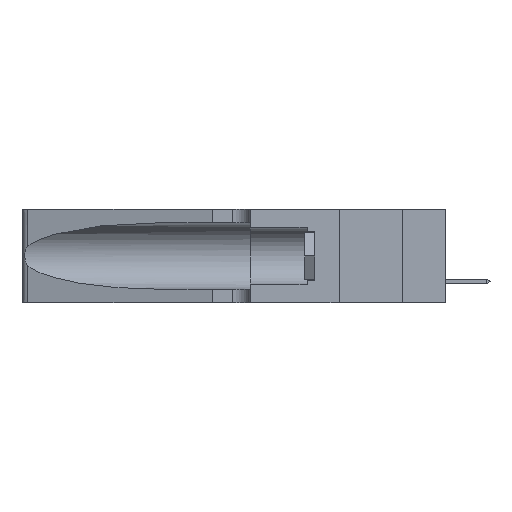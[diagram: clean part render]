
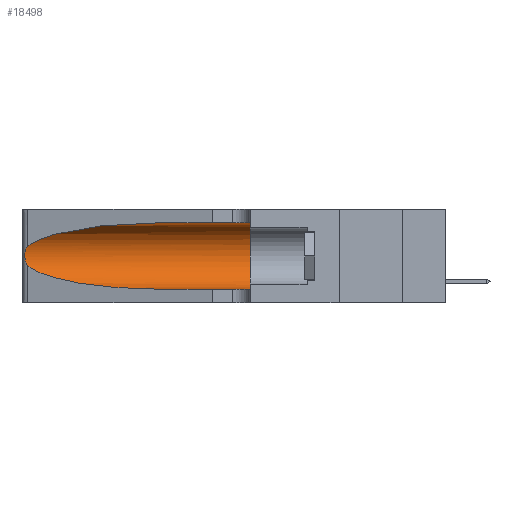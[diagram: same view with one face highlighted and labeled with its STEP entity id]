
A CAD part, left-side view. The second image highlights one B-rep face of the part: STEP entity #18498.
In plain terms, the highlighted cylindrical face has radius 3.308 mm (diameter 6.617 mm), a partial arc.
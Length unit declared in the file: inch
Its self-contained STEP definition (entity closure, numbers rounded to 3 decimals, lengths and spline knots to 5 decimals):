
#205 = EDGE_CURVE ( 'NONE', #29368, #12814, #3224, .T. ) ;
#414 = VERTEX_POINT ( 'NONE', #39376 ) ;
#607 = ORIENTED_EDGE ( 'NONE', *, *, #37022, .T. ) ;
#653 = DIRECTION ( 'NONE',  ( 0., -1., 0. ) ) ;
#864 = CARTESIAN_POINT ( 'NONE',  ( 0.1305, 0.72297, 0.05475 ) ) ;
#1577 = CARTESIAN_POINT ( 'NONE',  ( 0.1305, 1.61858, 0.185 ) ) ;
#1724 = DIRECTION ( 'NONE',  ( 0., 0., -1. ) ) ;
#2871 = EDGE_LOOP ( 'NONE', ( #3150, #14968, #9746, #607, #26021, #4308 ) ) ;
#2929 = CARTESIAN_POINT ( 'NONE',  ( 0.18966, 0.96281, 0.31525 ) ) ;
#3104 = CARTESIAN_POINT ( 'NONE',  ( 0.25555, 1.22994, 0.2215 ) ) ;
#3150 = ORIENTED_EDGE ( 'NONE', *, *, #29573, .T. ) ;
#3224 =( BOUNDED_CURVE ( )  B_SPLINE_CURVE ( 3, ( #22594, #19833, #13927, #26059 ),
 .UNSPECIFIED., .F., .T. ) 
 B_SPLINE_CURVE_WITH_KNOTS ( ( 4, 4 ),
 ( 3.44316, 4.71239 ),
 .UNSPECIFIED. ) 
 CURVE ( )  GEOMETRIC_REPRESENTATION_ITEM ( )  RATIONAL_B_SPLINE_CURVE ( ( 1., 0.87, 0.87, 1. ) ) 
 REPRESENTATION_ITEM ( '' )  );
#3244 = CARTESIAN_POINT ( 'NONE',  ( 0.25555, 1.22993, 0.14849 ) ) ;
#3361 = CARTESIAN_POINT ( 'NONE',  ( 0.25487, 1.22718, 0.14631 ) ) ;
#3392 = CARTESIAN_POINT ( 'NONE',  ( 0.1305, 1.61858, 0.05475 ) ) ;
#3402 = VERTEX_POINT ( 'NONE', #30428 ) ;
#4308 = ORIENTED_EDGE ( 'NONE', *, *, #9264, .F. ) ;
#4785 = CIRCLE ( 'NONE', #4884, 0.13025 ) ;
#4884 = AXIS2_PLACEMENT_3D ( 'NONE', #7861, #14032, #29852 ) ;
#5183 = FACE_OUTER_BOUND ( 'NONE', #2871, .T. ) ;
#5550 = DIRECTION ( 'NONE',  ( 0., -1., 0. ) ) ;
#6069 = CARTESIAN_POINT ( 'NONE',  ( 0.25487, 1.22718, 0.22369 ) ) ;
#6291 = EDGE_CURVE ( 'NONE', #3402, #29368, #35395, .T. ) ;
#7861 = CARTESIAN_POINT ( 'NONE',  ( 0.1305, 0.35, 0.185 ) ) ;
#9264 = EDGE_CURVE ( 'NONE', #22492, #414, #20604, .T. ) ;
#9746 = ORIENTED_EDGE ( 'NONE', *, *, #205, .T. ) ;
#12292 = VECTOR ( 'NONE', #653, 39.37008 ) ;
#12814 = VERTEX_POINT ( 'NONE', #864 ) ;
#12923 = CARTESIAN_POINT ( 'NONE',  ( 0.25639, 1.23186, 0.15144 ) ) ;
#13927 = CARTESIAN_POINT ( 'NONE',  ( 0.18966, 0.96281, 0.05475 ) ) ;
#13945 = EDGE_CURVE ( 'NONE', #414, #30024, #4785, .T. ) ;
#14032 = DIRECTION ( 'NONE',  ( 0., 1., 0. ) ) ;
#14605 = CARTESIAN_POINT ( 'NONE',  ( 0.25487, 1.22718, 0.14631 ) ) ;
#14890 = CARTESIAN_POINT ( 'NONE',  ( 0.26075, 1.23896, 0.19203 ) ) ;
#14968 = ORIENTED_EDGE ( 'NONE', *, *, #6291, .T. ) ;
#15111 = CARTESIAN_POINT ( 'NONE',  ( 0.25487, 1.22718, 0.22369 ) ) ;
#15850 = CARTESIAN_POINT ( 'NONE',  ( 0.25856, 1.23593, 0.16098 ) ) ;
#16203 = CARTESIAN_POINT ( 'NONE',  ( 0.1305, 0.72297, 0.31525 ) ) ;
#17083 =( BOUNDED_CURVE ( )  B_SPLINE_CURVE ( 3, ( #30319, #2929, #24384, #6069 ),
 .UNSPECIFIED., .F., .F. ) 
 B_SPLINE_CURVE_WITH_KNOTS ( ( 4, 4 ),
 ( 1.5708, 2.84003 ),
 .UNSPECIFIED. ) 
 CURVE ( )  GEOMETRIC_REPRESENTATION_ITEM ( )  RATIONAL_B_SPLINE_CURVE ( ( 1., 0.87, 0.87, 1. ) ) 
 REPRESENTATION_ITEM ( '' )  );
#17200 = CYLINDRICAL_SURFACE ( 'NONE', #24920, 0.13025 ) ;
#17259 = DIRECTION ( 'NONE',  ( 0., -1., 0. ) ) ;
#18498 = ADVANCED_FACE ( 'NONE', ( #5183 ), #17200, .F. ) ;
#19833 = CARTESIAN_POINT ( 'NONE',  ( 0.2373, 1.15595, 0.08982 ) ) ;
#20604 = LINE ( 'NONE', #28747, #31380 ) ;
#22017 = CARTESIAN_POINT ( 'NONE',  ( 0.25789, 1.23486, 0.15765 ) ) ;
#22255 = CARTESIAN_POINT ( 'NONE',  ( 0.25787, 1.23484, 0.2124 ) ) ;
#22492 = VERTEX_POINT ( 'NONE', #16203 ) ;
#22594 = CARTESIAN_POINT ( 'NONE',  ( 0.25487, 1.22718, 0.14631 ) ) ;
#24263 = LINE ( 'NONE', #3392, #12292 ) ;
#24384 = CARTESIAN_POINT ( 'NONE',  ( 0.2373, 1.15595, 0.28018 ) ) ;
#24920 = AXIS2_PLACEMENT_3D ( 'NONE', #1577, #5550, #1724 ) ;
#26021 = ORIENTED_EDGE ( 'NONE', *, *, #13945, .F. ) ;
#26059 = CARTESIAN_POINT ( 'NONE',  ( 0.1305, 0.72297, 0.05475 ) ) ;
#28063 = CARTESIAN_POINT ( 'NONE',  ( 0.1305, 0.35, 0.05475 ) ) ;
#28310 = CARTESIAN_POINT ( 'NONE',  ( 0.25854, 1.2359, 0.20912 ) ) ;
#28747 = CARTESIAN_POINT ( 'NONE',  ( 0.1305, 1.61858, 0.31525 ) ) ;
#29368 = VERTEX_POINT ( 'NONE', #14605 ) ;
#29573 = EDGE_CURVE ( 'NONE', #22492, #3402, #17083, .T. ) ;
#29852 = DIRECTION ( 'NONE',  ( 0., 0., 1. ) ) ;
#30024 = VERTEX_POINT ( 'NONE', #28063 ) ;
#30164 = CARTESIAN_POINT ( 'NONE',  ( 0.26017, 1.23833, 0.17102 ) ) ;
#30319 = CARTESIAN_POINT ( 'NONE',  ( 0.1305, 0.72297, 0.31525 ) ) ;
#30428 = CARTESIAN_POINT ( 'NONE',  ( 0.25487, 1.22718, 0.22369 ) ) ;
#30645 = CARTESIAN_POINT ( 'NONE',  ( 0.26018, 1.23835, 0.19895 ) ) ;
#31380 = VECTOR ( 'NONE', #17259, 39.37008 ) ;
#35395 = B_SPLINE_CURVE_WITH_KNOTS ( 'NONE', 3,
 ( #15111, #3104, #37000, #22255, #28310, #30645, #14890, #36234, #30164, #15850, #22017, #12923, #3244, #3361 ),
 .UNSPECIFIED., .F., .F.,
 ( 4, 2, 2, 2, 2, 2, 4 ),
 ( 0., 0.00027, 0.00053, 0.00107, 0.0016, 0.00187, 0.00214 ),
 .UNSPECIFIED. ) ;
#36234 = CARTESIAN_POINT ( 'NONE',  ( 0.26075, 1.23896, 0.178 ) ) ;
#37000 = CARTESIAN_POINT ( 'NONE',  ( 0.25639, 1.23184, 0.21858 ) ) ;
#37022 = EDGE_CURVE ( 'NONE', #12814, #30024, #24263, .T. ) ;
#39376 = CARTESIAN_POINT ( 'NONE',  ( 0.1305, 0.35, 0.31525 ) ) ;
